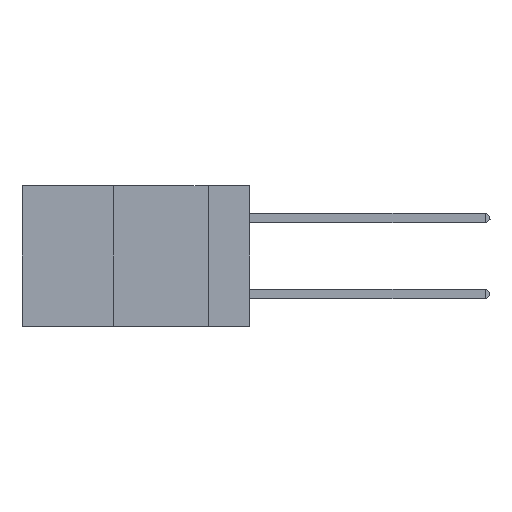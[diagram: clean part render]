
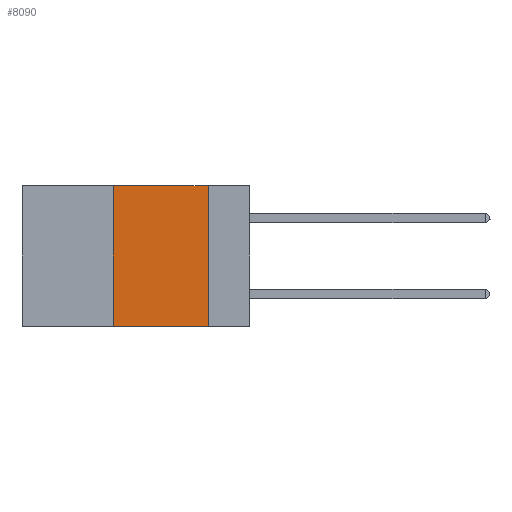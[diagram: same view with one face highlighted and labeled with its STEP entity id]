
A CAD part, left-side view. The second image highlights one B-rep face of the part: STEP entity #8090.
In plain terms, the highlighted planar face has unit normal (-1, 0, 0).
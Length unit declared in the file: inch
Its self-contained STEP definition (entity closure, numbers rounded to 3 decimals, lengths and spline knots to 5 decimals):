
#731 = VERTEX_POINT ( 'NONE', #8981 ) ;
#1128 = CARTESIAN_POINT ( 'NONE',  ( 0., 0.6, 0. ) ) ;
#1244 = FACE_OUTER_BOUND ( 'NONE', #7627, .T. ) ;
#1412 = LINE ( 'NONE', #14045, #12233 ) ;
#2462 = EDGE_CURVE ( 'NONE', #13234, #731, #1412, .T. ) ;
#3959 = DIRECTION ( 'NONE',  ( 0., 0., -1. ) ) ;
#4808 = EDGE_CURVE ( 'NONE', #13234, #7815, #8976, .T. ) ;
#5023 = LINE ( 'NONE', #1128, #15866 ) ;
#6061 = DIRECTION ( 'NONE',  ( 0., -1., 0. ) ) ;
#6132 = CARTESIAN_POINT ( 'NONE',  ( 0., 0.6, -0.37 ) ) ;
#6733 = CARTESIAN_POINT ( 'NONE',  ( 0., 0.11, -0.37 ) ) ;
#7627 = EDGE_LOOP ( 'NONE', ( #8793, #10063, #13923, #8714 ) ) ;
#7718 = EDGE_CURVE ( 'NONE', #8027, #7815, #14804, .T. ) ;
#7815 = VERTEX_POINT ( 'NONE', #6733 ) ;
#7899 = CARTESIAN_POINT ( 'NONE',  ( 0., 0.11, 0. ) ) ;
#8027 = VERTEX_POINT ( 'NONE', #7899 ) ;
#8090 = ADVANCED_FACE ( 'NONE', ( #1244 ), #10411, .F. ) ;
#8714 = ORIENTED_EDGE ( 'NONE', *, *, #4808, .T. ) ;
#8749 = VECTOR ( 'NONE', #12204, 39.37008 ) ;
#8793 = ORIENTED_EDGE ( 'NONE', *, *, #7718, .F. ) ;
#8976 = LINE ( 'NONE', #6132, #14055 ) ;
#8981 = CARTESIAN_POINT ( 'NONE',  ( 0., 0.36, 0. ) ) ;
#8989 = DIRECTION ( 'NONE',  ( 1., 0., 0. ) ) ;
#10063 = ORIENTED_EDGE ( 'NONE', *, *, #14597, .F. ) ;
#10239 = DIRECTION ( 'NONE',  ( 0., 0., 1. ) ) ;
#10411 = PLANE ( 'NONE',  #12596 ) ;
#11407 = DIRECTION ( 'NONE',  ( 0., -1., 0. ) ) ;
#11954 = CARTESIAN_POINT ( 'NONE',  ( 0., 0.11, 0. ) ) ;
#12204 = DIRECTION ( 'NONE',  ( 0., 0., -1. ) ) ;
#12233 = VECTOR ( 'NONE', #10239, 39.37008 ) ;
#12596 = AXIS2_PLACEMENT_3D ( 'NONE', #15551, #8989, #3959 ) ;
#12994 = CARTESIAN_POINT ( 'NONE',  ( 0., 0.36, -0.37 ) ) ;
#13234 = VERTEX_POINT ( 'NONE', #12994 ) ;
#13923 = ORIENTED_EDGE ( 'NONE', *, *, #2462, .F. ) ;
#14045 = CARTESIAN_POINT ( 'NONE',  ( 0., 0.36, 0. ) ) ;
#14055 = VECTOR ( 'NONE', #6061, 39.37008 ) ;
#14597 = EDGE_CURVE ( 'NONE', #731, #8027, #5023, .T. ) ;
#14804 = LINE ( 'NONE', #11954, #8749 ) ;
#15551 = CARTESIAN_POINT ( 'NONE',  ( 0., 0.6, 0. ) ) ;
#15866 = VECTOR ( 'NONE', #11407, 39.37008 ) ;
